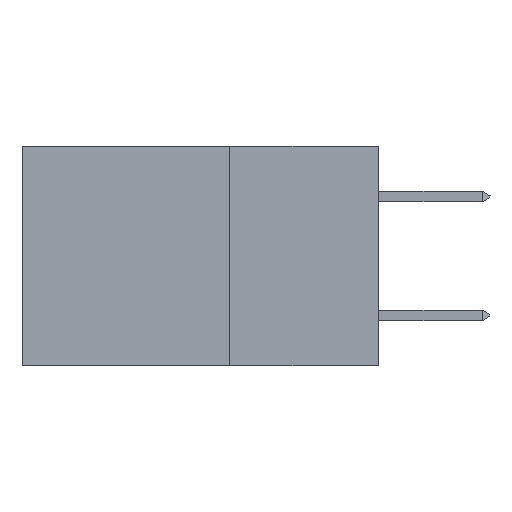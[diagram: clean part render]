
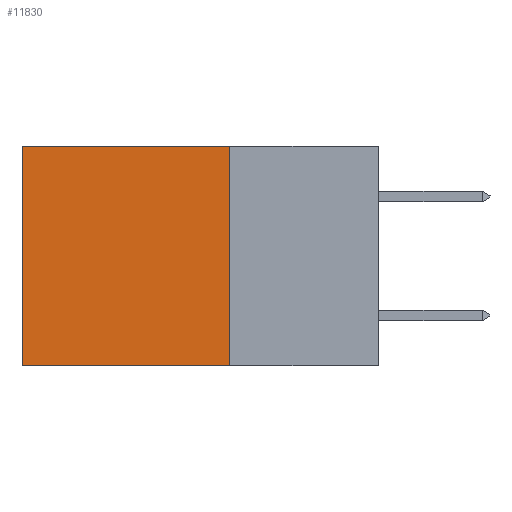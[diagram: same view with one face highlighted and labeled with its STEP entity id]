
A CAD part, left-side view. The second image highlights one B-rep face of the part: STEP entity #11830.
In plain terms, the highlighted planar face has unit normal (-1, 0, 0).
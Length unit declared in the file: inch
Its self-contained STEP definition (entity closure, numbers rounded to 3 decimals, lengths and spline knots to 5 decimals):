
#466 = DIRECTION ( 'NONE',  ( 0., 0., -1. ) ) ;
#565 = LINE ( 'NONE', #9077, #1783 ) ;
#859 = CARTESIAN_POINT ( 'NONE',  ( 0.2615, 0.6, -0.37 ) ) ;
#1157 = EDGE_CURVE ( 'NONE', #18522, #22904, #1518, .T. ) ;
#1518 = LINE ( 'NONE', #10036, #19324 ) ;
#1783 = VECTOR ( 'NONE', #24097, 39.37008 ) ;
#2343 = VECTOR ( 'NONE', #23540, 39.37008 ) ;
#4832 = PLANE ( 'NONE',  #9969 ) ;
#5117 = DIRECTION ( 'NONE',  ( 0., 0., -1. ) ) ;
#6362 = ORIENTED_EDGE ( 'NONE', *, *, #26702, .F. ) ;
#9077 = CARTESIAN_POINT ( 'NONE',  ( 0.2615, 0.6, -0.37 ) ) ;
#9969 = AXIS2_PLACEMENT_3D ( 'NONE', #24038, #13374, #5117 ) ;
#10036 = CARTESIAN_POINT ( 'NONE',  ( 0.2615, 0.25, 0. ) ) ;
#11830 = ADVANCED_FACE ( 'NONE', ( #22224 ), #4832, .F. ) ;
#12702 = EDGE_CURVE ( 'NONE', #27029, #17102, #23690, .T. ) ;
#13374 = DIRECTION ( 'NONE',  ( 1., 0., 0. ) ) ;
#14437 = ORIENTED_EDGE ( 'NONE', *, *, #1157, .T. ) ;
#16196 = VECTOR ( 'NONE', #466, 39.37008 ) ;
#16980 = EDGE_LOOP ( 'NONE', ( #26675, #25026, #6362, #14437 ) ) ;
#17102 = VERTEX_POINT ( 'NONE', #859 ) ;
#17437 = CARTESIAN_POINT ( 'NONE',  ( 0.2615, 0.6, 0. ) ) ;
#18045 = CARTESIAN_POINT ( 'NONE',  ( 0.2615, 0.25, -0.37 ) ) ;
#18522 = VERTEX_POINT ( 'NONE', #21917 ) ;
#19324 = VECTOR ( 'NONE', #25063, 39.37008 ) ;
#19664 = CARTESIAN_POINT ( 'NONE',  ( 0.2615, 0.25, -0.37 ) ) ;
#21917 = CARTESIAN_POINT ( 'NONE',  ( 0.2615, 0.25, 0. ) ) ;
#22224 = FACE_OUTER_BOUND ( 'NONE', #16980, .T. ) ;
#22318 = LINE ( 'NONE', #19664, #16196 ) ;
#22904 = VERTEX_POINT ( 'NONE', #17437 ) ;
#23540 = DIRECTION ( 'NONE',  ( 0., 1., 0. ) ) ;
#23690 = LINE ( 'NONE', #18045, #2343 ) ;
#24038 = CARTESIAN_POINT ( 'NONE',  ( 0.2615, 0.25, -0.37 ) ) ;
#24097 = DIRECTION ( 'NONE',  ( 0., 0., -1. ) ) ;
#24111 = EDGE_CURVE ( 'NONE', #22904, #17102, #565, .T. ) ;
#25026 = ORIENTED_EDGE ( 'NONE', *, *, #12702, .F. ) ;
#25063 = DIRECTION ( 'NONE',  ( 0., 1., 0. ) ) ;
#26192 = CARTESIAN_POINT ( 'NONE',  ( 0.2615, 0.25, -0.37 ) ) ;
#26675 = ORIENTED_EDGE ( 'NONE', *, *, #24111, .T. ) ;
#26702 = EDGE_CURVE ( 'NONE', #18522, #27029, #22318, .T. ) ;
#27029 = VERTEX_POINT ( 'NONE', #26192 ) ;
